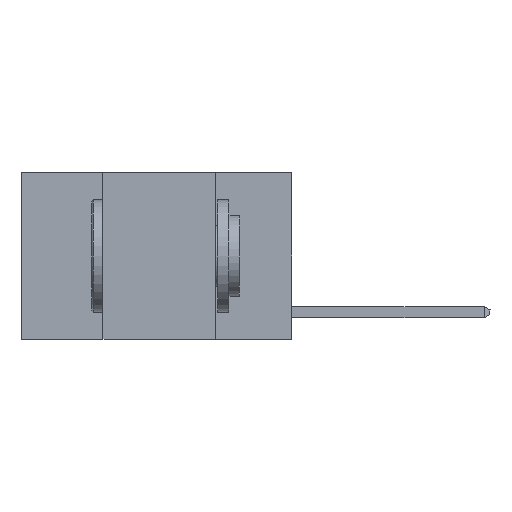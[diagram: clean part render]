
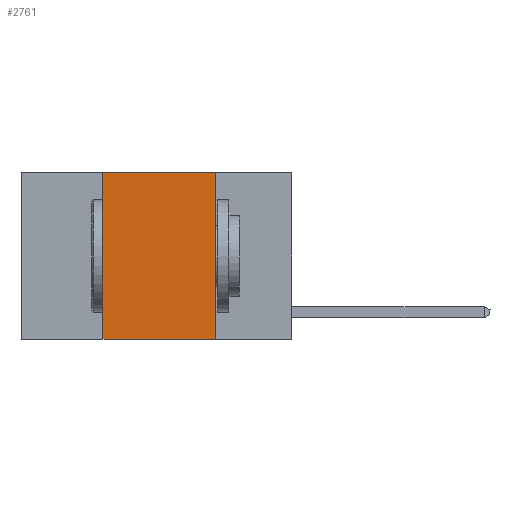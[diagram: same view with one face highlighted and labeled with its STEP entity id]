
A CAD part, left-side view. The second image highlights one B-rep face of the part: STEP entity #2761.
In plain terms, the highlighted planar face has unit normal (-1, 0, 0).
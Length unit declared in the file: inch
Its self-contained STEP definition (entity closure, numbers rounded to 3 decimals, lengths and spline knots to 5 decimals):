
#472 = VERTEX_POINT ( 'NONE', #5766 ) ;
#644 = LINE ( 'NONE', #2106, #6024 ) ;
#1357 = VERTEX_POINT ( 'NONE', #4106 ) ;
#1717 = CARTESIAN_POINT ( 'NONE',  ( 0., 0.17, 0. ) ) ;
#2106 = CARTESIAN_POINT ( 'NONE',  ( 0., 0.6, -0.37 ) ) ;
#2211 = ORIENTED_EDGE ( 'NONE', *, *, #6914, .T. ) ;
#2761 = ADVANCED_FACE ( 'NONE', ( #6213 ), #4440, .F. ) ;
#2831 = CARTESIAN_POINT ( 'NONE',  ( 0., 0.42, 0. ) ) ;
#4106 = CARTESIAN_POINT ( 'NONE',  ( 0., 0.42, -0.37 ) ) ;
#4440 = PLANE ( 'NONE',  #9204 ) ;
#4695 = EDGE_CURVE ( 'NONE', #11035, #472, #4845, .T. ) ;
#4708 = CARTESIAN_POINT ( 'NONE',  ( 0., 0.6, 0. ) ) ;
#4845 = LINE ( 'NONE', #4708, #12195 ) ;
#5274 = CARTESIAN_POINT ( 'NONE',  ( 0., 0.42, 0. ) ) ;
#5766 = CARTESIAN_POINT ( 'NONE',  ( 0., 0.17, 0. ) ) ;
#6024 = VECTOR ( 'NONE', #10276, 39.37008 ) ;
#6213 = FACE_OUTER_BOUND ( 'NONE', #12990, .T. ) ;
#6555 = DIRECTION ( 'NONE',  ( 0., 0., -1. ) ) ;
#6673 = EDGE_CURVE ( 'NONE', #472, #11640, #8852, .T. ) ;
#6828 = VECTOR ( 'NONE', #8967, 39.37008 ) ;
#6914 = EDGE_CURVE ( 'NONE', #1357, #11640, #644, .T. ) ;
#7116 = ORIENTED_EDGE ( 'NONE', *, *, #6673, .F. ) ;
#7421 = ORIENTED_EDGE ( 'NONE', *, *, #8244, .F. ) ;
#7878 = VECTOR ( 'NONE', #7984, 39.37008 ) ;
#7984 = DIRECTION ( 'NONE',  ( 0., 0., 1. ) ) ;
#8182 = LINE ( 'NONE', #2831, #7878 ) ;
#8244 = EDGE_CURVE ( 'NONE', #1357, #11035, #8182, .T. ) ;
#8852 = LINE ( 'NONE', #1717, #6828 ) ;
#8967 = DIRECTION ( 'NONE',  ( 0., 0., -1. ) ) ;
#9204 = AXIS2_PLACEMENT_3D ( 'NONE', #11484, #12449, #6555 ) ;
#9752 = ORIENTED_EDGE ( 'NONE', *, *, #4695, .F. ) ;
#10276 = DIRECTION ( 'NONE',  ( 0., -1., 0. ) ) ;
#11035 = VERTEX_POINT ( 'NONE', #5274 ) ;
#11484 = CARTESIAN_POINT ( 'NONE',  ( 0., 0.6, 0. ) ) ;
#11640 = VERTEX_POINT ( 'NONE', #12014 ) ;
#12014 = CARTESIAN_POINT ( 'NONE',  ( 0., 0.17, -0.37 ) ) ;
#12195 = VECTOR ( 'NONE', #12694, 39.37008 ) ;
#12449 = DIRECTION ( 'NONE',  ( 1., 0., 0. ) ) ;
#12694 = DIRECTION ( 'NONE',  ( 0., -1., 0. ) ) ;
#12990 = EDGE_LOOP ( 'NONE', ( #7116, #9752, #7421, #2211 ) ) ;
